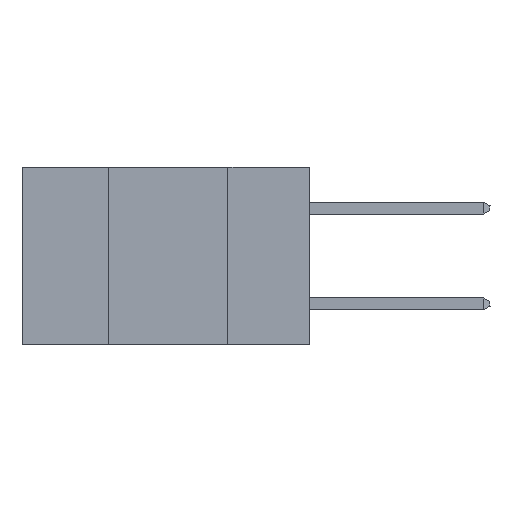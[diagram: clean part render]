
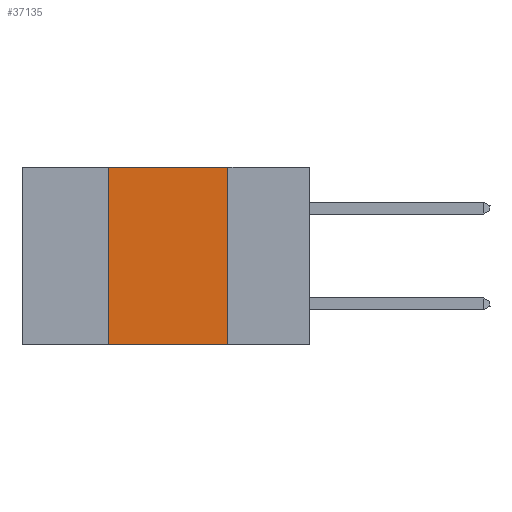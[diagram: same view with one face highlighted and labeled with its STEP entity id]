
A CAD part, left-side view. The second image highlights one B-rep face of the part: STEP entity #37135.
In plain terms, the highlighted planar face has unit normal (-1, 0, 0).
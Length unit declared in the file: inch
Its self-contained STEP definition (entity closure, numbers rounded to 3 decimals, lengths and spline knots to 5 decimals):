
#989 = CARTESIAN_POINT ( 'NONE',  ( 0., 0.6, 0. ) ) ;
#2590 = ORIENTED_EDGE ( 'NONE', *, *, #2671, .F. ) ;
#2671 = EDGE_CURVE ( 'NONE', #25128, #9748, #17588, .T. ) ;
#2773 = CARTESIAN_POINT ( 'NONE',  ( 0., 0.17, 0. ) ) ;
#3016 = ORIENTED_EDGE ( 'NONE', *, *, #36428, .T. ) ;
#4425 = DIRECTION ( 'NONE',  ( 1., 0., 0. ) ) ;
#4481 = DIRECTION ( 'NONE',  ( 0., -1., 0. ) ) ;
#4567 = CARTESIAN_POINT ( 'NONE',  ( 0., 0.6, 0. ) ) ;
#4701 = EDGE_LOOP ( 'NONE', ( #27087, #31036, #2590, #3016 ) ) ;
#4968 = VECTOR ( 'NONE', #20950, 39.37008 ) ;
#6544 = CARTESIAN_POINT ( 'NONE',  ( 0., 0.42, 0. ) ) ;
#7277 = CARTESIAN_POINT ( 'NONE',  ( 0., 0.6, -0.37 ) ) ;
#7749 = VERTEX_POINT ( 'NONE', #23986 ) ;
#9202 = EDGE_CURVE ( 'NONE', #9748, #7749, #15713, .T. ) ;
#9748 = VERTEX_POINT ( 'NONE', #6544 ) ;
#12777 = DIRECTION ( 'NONE',  ( 0., 0., -1. ) ) ;
#15188 = VECTOR ( 'NONE', #17415, 39.37008 ) ;
#15713 = LINE ( 'NONE', #989, #32455 ) ;
#17225 = CARTESIAN_POINT ( 'NONE',  ( 0., 0.42, 0. ) ) ;
#17415 = DIRECTION ( 'NONE',  ( 0., 0., -1. ) ) ;
#17588 = LINE ( 'NONE', #17225, #4968 ) ;
#20950 = DIRECTION ( 'NONE',  ( 0., 0., 1. ) ) ;
#23387 = EDGE_CURVE ( 'NONE', #7749, #26208, #26920, .T. ) ;
#23749 = FACE_OUTER_BOUND ( 'NONE', #4701, .T. ) ;
#23986 = CARTESIAN_POINT ( 'NONE',  ( 0., 0.17, 0. ) ) ;
#24363 = DIRECTION ( 'NONE',  ( 0., -1., 0. ) ) ;
#24885 = PLANE ( 'NONE',  #35233 ) ;
#25128 = VERTEX_POINT ( 'NONE', #29003 ) ;
#26208 = VERTEX_POINT ( 'NONE', #33903 ) ;
#26920 = LINE ( 'NONE', #2773, #15188 ) ;
#27087 = ORIENTED_EDGE ( 'NONE', *, *, #23387, .F. ) ;
#28375 = VECTOR ( 'NONE', #4481, 39.37008 ) ;
#29003 = CARTESIAN_POINT ( 'NONE',  ( 0., 0.42, -0.37 ) ) ;
#31036 = ORIENTED_EDGE ( 'NONE', *, *, #9202, .F. ) ;
#32455 = VECTOR ( 'NONE', #24363, 39.37008 ) ;
#33390 = LINE ( 'NONE', #7277, #28375 ) ;
#33903 = CARTESIAN_POINT ( 'NONE',  ( 0., 0.17, -0.37 ) ) ;
#35233 = AXIS2_PLACEMENT_3D ( 'NONE', #4567, #4425, #12777 ) ;
#36428 = EDGE_CURVE ( 'NONE', #25128, #26208, #33390, .T. ) ;
#37135 = ADVANCED_FACE ( 'NONE', ( #23749 ), #24885, .F. ) ;
